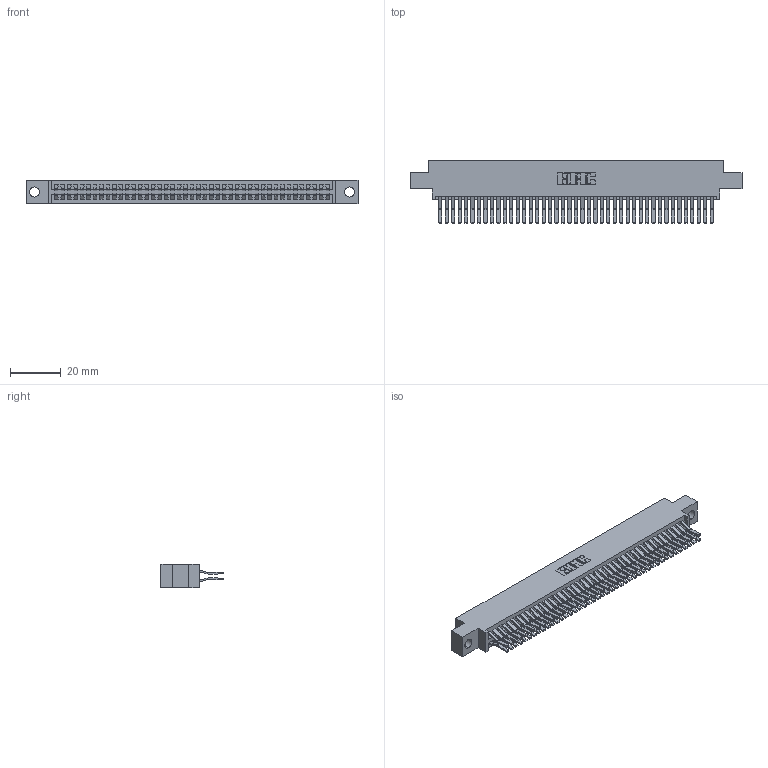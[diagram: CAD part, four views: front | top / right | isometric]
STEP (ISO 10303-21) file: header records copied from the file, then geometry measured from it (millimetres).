
FILE_DESCRIPTION (( 'STEP AP203' ), '1' );
FILE_NAME ('395-086-560-804.STEP', '2021-06-17T09:15:04', ( '' ), ( '' ), 'SwSTEP 2.0', 'SolidWorks 2020', '' );
FILE_SCHEMA (( 'CONFIG_CONTROL_DESIGN' ));
Length unit declared in the file: inch
Products named in the file (3): 345 Part_0.170 Offset - 0.156 Dia-TI; 345-292-001_560 Tail; 395-086-560-804
Assembly tree (87 placements, depth 2):
  395-086-560-804
    345 Part_0.170 Offset - 0.156 Dia-TI
    345-292-001_560 Tail  x86
Bounding box: 130.43 x 24.45 x 9.4 mm (x, y, z)
Volume: 13023.7 mm3; surface area: 20715.3 mm2
Topology: 87 solids, 87 shells, 4616 faces, 13719 edges, 9030 vertices
Faces by surface type: plane 2936, cylinder 1680
Entity records: 34243 total; most frequent: CARTESIAN_POINT 5746, ORIENTED_EDGE 5678, DIRECTION 5067, EDGE_CURVE 2839, LINE 2531, VECTOR 2531, VERTEX_POINT 1890, AXIS2_PLACEMENT_3D 1268
